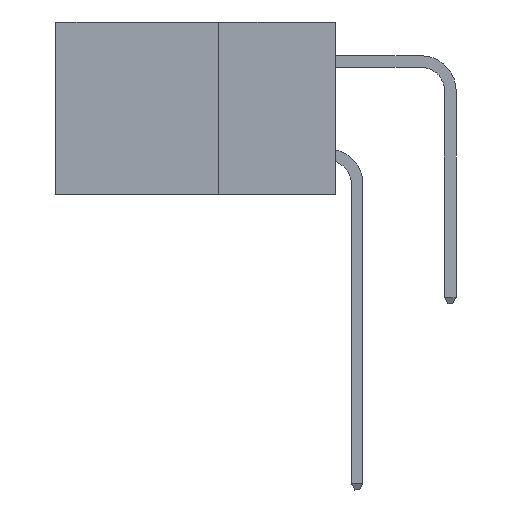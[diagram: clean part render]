
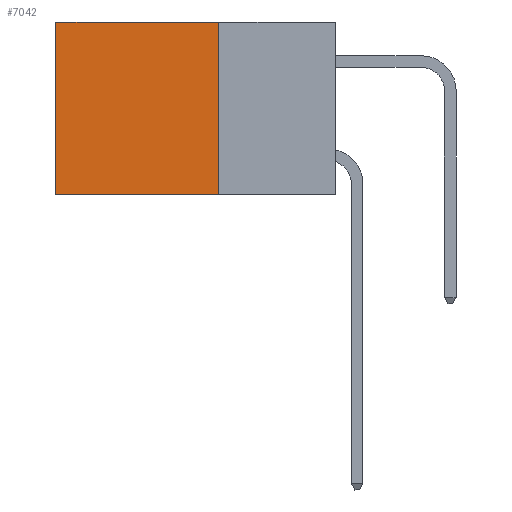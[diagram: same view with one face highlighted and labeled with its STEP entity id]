
A CAD part, left-side view. The second image highlights one B-rep face of the part: STEP entity #7042.
In plain terms, the highlighted planar face has unit normal (-1, 0, 0).
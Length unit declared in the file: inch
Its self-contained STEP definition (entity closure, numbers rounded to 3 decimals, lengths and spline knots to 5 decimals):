
#771 = CARTESIAN_POINT ( 'NONE',  ( 0.2875, 0.25, 0. ) ) ;
#899 = DIRECTION ( 'NONE',  ( 0., 0., -1. ) ) ;
#1101 = CARTESIAN_POINT ( 'NONE',  ( 0.2875, 0.25, 0. ) ) ;
#1602 = VERTEX_POINT ( 'NONE', #16983 ) ;
#1619 = ORIENTED_EDGE ( 'NONE', *, *, #4368, .F. ) ;
#2334 = LINE ( 'NONE', #8647, #17136 ) ;
#2356 = DIRECTION ( 'NONE',  ( 0., 0., -1. ) ) ;
#2432 = EDGE_CURVE ( 'NONE', #16311, #14323, #12077, .T. ) ;
#3040 = VECTOR ( 'NONE', #10540, 39.37008 ) ;
#3066 = CARTESIAN_POINT ( 'NONE',  ( 0.2875, 0.25, 0. ) ) ;
#4368 = EDGE_CURVE ( 'NONE', #16311, #14198, #9831, .T. ) ;
#5818 = ORIENTED_EDGE ( 'NONE', *, *, #2432, .T. ) ;
#5884 = AXIS2_PLACEMENT_3D ( 'NONE', #1101, #17994, #899 ) ;
#6323 = EDGE_LOOP ( 'NONE', ( #18011, #9005, #1619, #5818 ) ) ;
#6953 = CARTESIAN_POINT ( 'NONE',  ( 0.2875, 0.6, 0. ) ) ;
#7042 = ADVANCED_FACE ( 'NONE', ( #14855 ), #8541, .F. ) ;
#7214 = DIRECTION ( 'NONE',  ( 0., 1., 0. ) ) ;
#7283 = VECTOR ( 'NONE', #8408, 39.37008 ) ;
#8298 = EDGE_CURVE ( 'NONE', #14198, #1602, #2334, .T. ) ;
#8408 = DIRECTION ( 'NONE',  ( 0., 0., -1. ) ) ;
#8541 = PLANE ( 'NONE',  #5884 ) ;
#8647 = CARTESIAN_POINT ( 'NONE',  ( 0.2875, 0.25, -0.37 ) ) ;
#8778 = EDGE_CURVE ( 'NONE', #14323, #1602, #17726, .T. ) ;
#9005 = ORIENTED_EDGE ( 'NONE', *, *, #8298, .F. ) ;
#9518 = CARTESIAN_POINT ( 'NONE',  ( 0.2875, 0.25, -0.37 ) ) ;
#9831 = LINE ( 'NONE', #771, #7283 ) ;
#10540 = DIRECTION ( 'NONE',  ( 0., 1., 0. ) ) ;
#10804 = VECTOR ( 'NONE', #2356, 39.37008 ) ;
#12077 = LINE ( 'NONE', #15326, #3040 ) ;
#14198 = VERTEX_POINT ( 'NONE', #9518 ) ;
#14323 = VERTEX_POINT ( 'NONE', #14907 ) ;
#14855 = FACE_OUTER_BOUND ( 'NONE', #6323, .T. ) ;
#14907 = CARTESIAN_POINT ( 'NONE',  ( 0.2875, 0.6, 0. ) ) ;
#15326 = CARTESIAN_POINT ( 'NONE',  ( 0.2875, 0.25, 0. ) ) ;
#16311 = VERTEX_POINT ( 'NONE', #3066 ) ;
#16983 = CARTESIAN_POINT ( 'NONE',  ( 0.2875, 0.6, -0.37 ) ) ;
#17136 = VECTOR ( 'NONE', #7214, 39.37008 ) ;
#17726 = LINE ( 'NONE', #6953, #10804 ) ;
#17994 = DIRECTION ( 'NONE',  ( 1., 0., 0. ) ) ;
#18011 = ORIENTED_EDGE ( 'NONE', *, *, #8778, .T. ) ;
